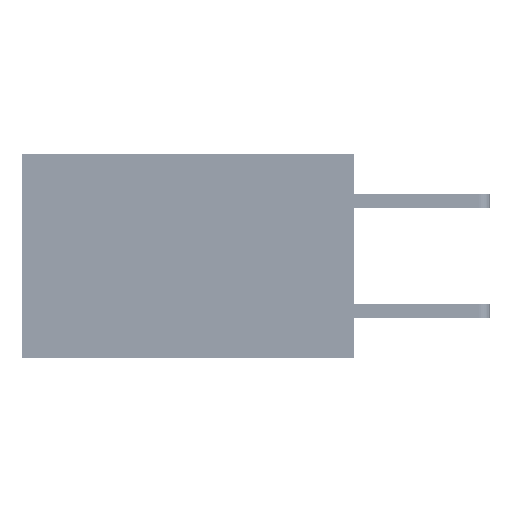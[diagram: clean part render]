
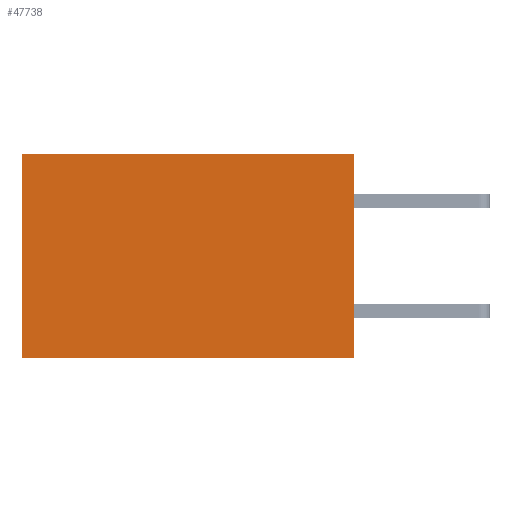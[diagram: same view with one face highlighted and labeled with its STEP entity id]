
A CAD part, left-side view. The second image highlights one B-rep face of the part: STEP entity #47738.
In plain terms, the highlighted planar face has unit normal (-1, 0, 0).
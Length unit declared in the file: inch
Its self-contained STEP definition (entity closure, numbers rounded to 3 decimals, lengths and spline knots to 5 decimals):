
#588 = ORIENTED_EDGE ( 'NONE', *, *, #20383, .T. ) ;
#790 = LINE ( 'NONE', #39099, #31719 ) ;
#1174 = DIRECTION ( 'NONE',  ( 0., 0., -1. ) ) ;
#1531 = CARTESIAN_POINT ( 'NONE',  ( 0.2875, 0.6, 0. ) ) ;
#2579 = ORIENTED_EDGE ( 'NONE', *, *, #47726, .T. ) ;
#5889 = VECTOR ( 'NONE', #13157, 39.37008 ) ;
#6016 = DIRECTION ( 'NONE',  ( 0., 1., 0. ) ) ;
#6539 = CARTESIAN_POINT ( 'NONE',  ( 0.2875, 0., -0.37 ) ) ;
#8316 = CARTESIAN_POINT ( 'NONE',  ( 0.2875, 0.6, 0. ) ) ;
#8550 = DIRECTION ( 'NONE',  ( 0., 0., -1. ) ) ;
#9679 = ORIENTED_EDGE ( 'NONE', *, *, #33859, .F. ) ;
#9680 = DIRECTION ( 'NONE',  ( 1., 0., 0. ) ) ;
#9718 = CARTESIAN_POINT ( 'NONE',  ( 0.2875, 0., -0.37 ) ) ;
#10176 = ORIENTED_EDGE ( 'NONE', *, *, #38086, .F. ) ;
#13157 = DIRECTION ( 'NONE',  ( 0., 0., -1. ) ) ;
#14357 = CARTESIAN_POINT ( 'NONE',  ( 0.2875, 0., 0. ) ) ;
#16587 = LINE ( 'NONE', #1531, #5889 ) ;
#18417 = VERTEX_POINT ( 'NONE', #9718 ) ;
#20383 = EDGE_CURVE ( 'NONE', #37700, #32120, #790, .T. ) ;
#26482 = VECTOR ( 'NONE', #6016, 39.37008 ) ;
#29886 = CARTESIAN_POINT ( 'NONE',  ( 0.2875, 0.6, -0.37 ) ) ;
#31719 = VECTOR ( 'NONE', #46994, 39.37008 ) ;
#32120 = VERTEX_POINT ( 'NONE', #8316 ) ;
#32684 = CARTESIAN_POINT ( 'NONE',  ( 0.2875, 0., 0. ) ) ;
#33774 = PLANE ( 'NONE',  #36308 ) ;
#33859 = EDGE_CURVE ( 'NONE', #18417, #51433, #47849, .T. ) ;
#36308 = AXIS2_PLACEMENT_3D ( 'NONE', #45390, #9680, #1174 ) ;
#37700 = VERTEX_POINT ( 'NONE', #14357 ) ;
#38086 = EDGE_CURVE ( 'NONE', #37700, #18417, #51434, .T. ) ;
#39099 = CARTESIAN_POINT ( 'NONE',  ( 0.2875, 0., 0. ) ) ;
#43652 = EDGE_LOOP ( 'NONE', ( #2579, #9679, #10176, #588 ) ) ;
#45390 = CARTESIAN_POINT ( 'NONE',  ( 0.2875, 0., 0. ) ) ;
#46994 = DIRECTION ( 'NONE',  ( 0., 1., 0. ) ) ;
#47462 = FACE_OUTER_BOUND ( 'NONE', #43652, .T. ) ;
#47726 = EDGE_CURVE ( 'NONE', #32120, #51433, #16587, .T. ) ;
#47738 = ADVANCED_FACE ( 'NONE', ( #47462 ), #33774, .F. ) ;
#47849 = LINE ( 'NONE', #6539, #26482 ) ;
#49562 = VECTOR ( 'NONE', #8550, 39.37008 ) ;
#51433 = VERTEX_POINT ( 'NONE', #29886 ) ;
#51434 = LINE ( 'NONE', #32684, #49562 ) ;
